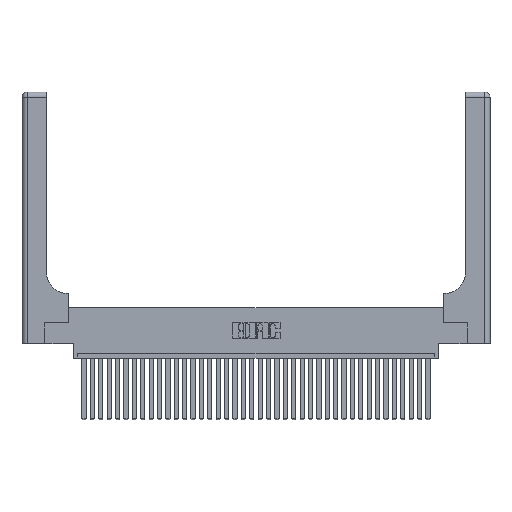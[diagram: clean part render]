
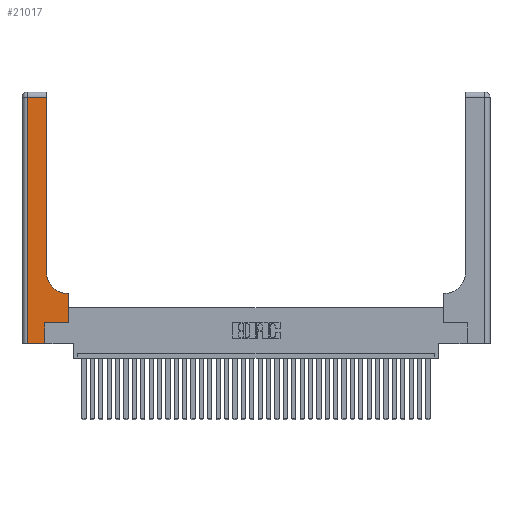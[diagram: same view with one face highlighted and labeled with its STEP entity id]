
A CAD part, top view. The second image highlights one B-rep face of the part: STEP entity #21017.
In plain terms, the highlighted planar face has unit normal (0, 0, 1).
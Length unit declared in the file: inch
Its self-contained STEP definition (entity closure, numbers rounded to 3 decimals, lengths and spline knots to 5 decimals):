
#217 = CARTESIAN_POINT ( 'NONE',  ( 0.2915, 0.85, 0.37 ) ) ;
#613 = DIRECTION ( 'NONE',  ( 0., 1., 0. ) ) ;
#996 = CARTESIAN_POINT ( 'NONE',  ( 0.269, 0., 0.37 ) ) ;
#1906 = VERTEX_POINT ( 'NONE', #16095 ) ;
#1907 = EDGE_CURVE ( 'NONE', #12921, #1906, #32813, .T. ) ;
#1940 = VERTEX_POINT ( 'NONE', #30961 ) ;
#2386 = ORIENTED_EDGE ( 'NONE', *, *, #11488, .T. ) ;
#2610 = CARTESIAN_POINT ( 'NONE',  ( 0., 2.94, 0.37 ) ) ;
#3373 = CARTESIAN_POINT ( 'NONE',  ( 0.2915, 3., 0.37 ) ) ;
#3559 = LINE ( 'NONE', #996, #25322 ) ;
#3611 = DIRECTION ( 'NONE',  ( 0., 0., -1. ) ) ;
#4673 = CARTESIAN_POINT ( 'NONE',  ( 0.5415, 0.85, 0.37 ) ) ;
#5482 = DIRECTION ( 'NONE',  ( 0., -1., 0. ) ) ;
#5844 = EDGE_LOOP ( 'NONE', ( #34147, #2386, #26236, #27153, #13915, #23630, #14284, #34112, #8031 ) ) ;
#6132 = VECTOR ( 'NONE', #22076, 39.37008 ) ;
#6447 = CARTESIAN_POINT ( 'NONE',  ( 0.269, 0.25, 0.37 ) ) ;
#7782 = EDGE_CURVE ( 'NONE', #9935, #19363, #13931, .T. ) ;
#8031 = ORIENTED_EDGE ( 'NONE', *, *, #10131, .T. ) ;
#8066 = FACE_OUTER_BOUND ( 'NONE', #5844, .T. ) ;
#9935 = VERTEX_POINT ( 'NONE', #27839 ) ;
#10131 = EDGE_CURVE ( 'NONE', #19363, #26039, #26181, .T. ) ;
#10363 = VECTOR ( 'NONE', #12199, 39.37008 ) ;
#10719 = CARTESIAN_POINT ( 'NONE',  ( 0.2915, 2.94, 0.37 ) ) ;
#11488 = EDGE_CURVE ( 'NONE', #32629, #31267, #25212, .T. ) ;
#11660 = CARTESIAN_POINT ( 'NONE',  ( 0., 3., 0.37 ) ) ;
#12199 = DIRECTION ( 'NONE',  ( -1., 0., 0. ) ) ;
#12443 = CARTESIAN_POINT ( 'NONE',  ( 0.06, 2.94, 0.37 ) ) ;
#12921 = VERTEX_POINT ( 'NONE', #17807 ) ;
#13915 = ORIENTED_EDGE ( 'NONE', *, *, #21223, .T. ) ;
#13931 = LINE ( 'NONE', #23242, #10363 ) ;
#14284 = ORIENTED_EDGE ( 'NONE', *, *, #34032, .T. ) ;
#14613 = LINE ( 'NONE', #22533, #17278 ) ;
#14682 = VECTOR ( 'NONE', #5482, 39.37008 ) ;
#15473 = EDGE_CURVE ( 'NONE', #31267, #12921, #22284, .T. ) ;
#15526 = LINE ( 'NONE', #6447, #19576 ) ;
#16095 = CARTESIAN_POINT ( 'NONE',  ( 0.269, 0., 0.37 ) ) ;
#16345 = CARTESIAN_POINT ( 'NONE',  ( 0., 0., 0.37 ) ) ;
#17278 = VECTOR ( 'NONE', #36546, 39.37008 ) ;
#17717 = VECTOR ( 'NONE', #27786, 39.37008 ) ;
#17807 = CARTESIAN_POINT ( 'NONE',  ( 0.06, 0., 0.37 ) ) ;
#17832 = CARTESIAN_POINT ( 'NONE',  ( 0.5415, 0.6, 0.37 ) ) ;
#18485 = DIRECTION ( 'NONE',  ( 0., 1., 0. ) ) ;
#19363 = VERTEX_POINT ( 'NONE', #17832 ) ;
#19576 = VECTOR ( 'NONE', #31930, 39.37008 ) ;
#21017 = ADVANCED_FACE ( 'NONE', ( #8066 ), #34586, .F. ) ;
#21223 = EDGE_CURVE ( 'NONE', #1906, #32247, #3559, .T. ) ;
#22076 = DIRECTION ( 'NONE',  ( -1., 0., 0. ) ) ;
#22284 = LINE ( 'NONE', #33204, #14682 ) ;
#22533 = CARTESIAN_POINT ( 'NONE',  ( 0.5585, 0.25, 0.37 ) ) ;
#23242 = CARTESIAN_POINT ( 'NONE',  ( 0.2915, 0.6, 0.37 ) ) ;
#23630 = ORIENTED_EDGE ( 'NONE', *, *, #26086, .T. ) ;
#25212 = LINE ( 'NONE', #2610, #6132 ) ;
#25322 = VECTOR ( 'NONE', #18485, 39.37008 ) ;
#25339 = AXIS2_PLACEMENT_3D ( 'NONE', #4673, #26822, #27332 ) ;
#25973 = CARTESIAN_POINT ( 'NONE',  ( 0.269, 0.25, 0.37 ) ) ;
#26039 = VERTEX_POINT ( 'NONE', #217 ) ;
#26086 = EDGE_CURVE ( 'NONE', #32247, #1940, #15526, .T. ) ;
#26181 = CIRCLE ( 'NONE', #25339, 0.25 ) ;
#26236 = ORIENTED_EDGE ( 'NONE', *, *, #15473, .T. ) ;
#26822 = DIRECTION ( 'NONE',  ( 0., 0., -1. ) ) ;
#27153 = ORIENTED_EDGE ( 'NONE', *, *, #1907, .T. ) ;
#27332 = DIRECTION ( 'NONE',  ( 1., 0., 0. ) ) ;
#27786 = DIRECTION ( 'NONE',  ( 1., 0., 0. ) ) ;
#27839 = CARTESIAN_POINT ( 'NONE',  ( 0.5585, 0.6, 0.37 ) ) ;
#28670 = AXIS2_PLACEMENT_3D ( 'NONE', #11660, #3611, #31464 ) ;
#30961 = CARTESIAN_POINT ( 'NONE',  ( 0.5585, 0.25, 0.37 ) ) ;
#31267 = VERTEX_POINT ( 'NONE', #12443 ) ;
#31464 = DIRECTION ( 'NONE',  ( -1., 0., 0. ) ) ;
#31930 = DIRECTION ( 'NONE',  ( 1., 0., 0. ) ) ;
#32247 = VERTEX_POINT ( 'NONE', #25973 ) ;
#32629 = VERTEX_POINT ( 'NONE', #10719 ) ;
#32813 = LINE ( 'NONE', #16345, #17717 ) ;
#32817 = EDGE_CURVE ( 'NONE', #26039, #32629, #33820, .T. ) ;
#32906 = VECTOR ( 'NONE', #613, 39.37008 ) ;
#33204 = CARTESIAN_POINT ( 'NONE',  ( 0.06, 3., 0.37 ) ) ;
#33820 = LINE ( 'NONE', #3373, #32906 ) ;
#34032 = EDGE_CURVE ( 'NONE', #1940, #9935, #14613, .T. ) ;
#34112 = ORIENTED_EDGE ( 'NONE', *, *, #7782, .T. ) ;
#34147 = ORIENTED_EDGE ( 'NONE', *, *, #32817, .T. ) ;
#34586 = PLANE ( 'NONE',  #28670 ) ;
#36546 = DIRECTION ( 'NONE',  ( 0., 1., 0. ) ) ;
